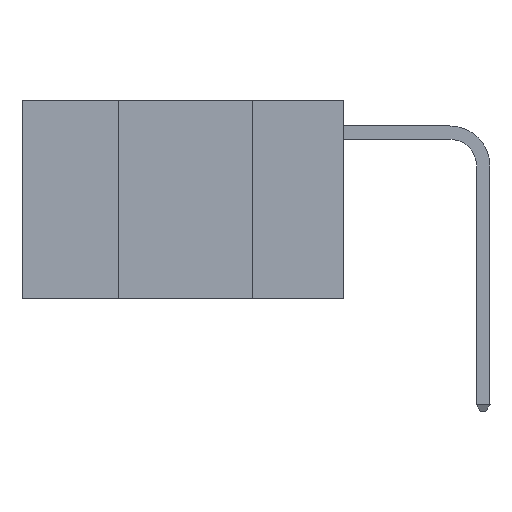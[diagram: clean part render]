
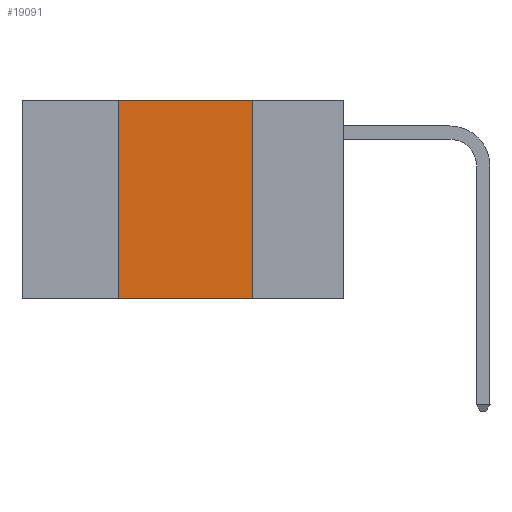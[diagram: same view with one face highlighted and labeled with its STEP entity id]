
A CAD part, left-side view. The second image highlights one B-rep face of the part: STEP entity #19091.
In plain terms, the highlighted planar face has unit normal (-1, 0, 0).
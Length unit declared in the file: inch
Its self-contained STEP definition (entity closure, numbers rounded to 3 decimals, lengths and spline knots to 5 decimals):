
#1354 = CARTESIAN_POINT ( 'NONE',  ( 0., 0.6, 0. ) ) ;
#1694 = CARTESIAN_POINT ( 'NONE',  ( 0., 0.17, 0. ) ) ;
#1809 = AXIS2_PLACEMENT_3D ( 'NONE', #28655, #1908, #17654 ) ;
#1908 = DIRECTION ( 'NONE',  ( 1., 0., 0. ) ) ;
#2780 = VERTEX_POINT ( 'NONE', #6010 ) ;
#4047 = ORIENTED_EDGE ( 'NONE', *, *, #19208, .T. ) ;
#4631 = DIRECTION ( 'NONE',  ( 0., -1., 0. ) ) ;
#4826 = EDGE_CURVE ( 'NONE', #10101, #12527, #15835, .T. ) ;
#5591 = EDGE_CURVE ( 'NONE', #12527, #10860, #24481, .T. ) ;
#6010 = CARTESIAN_POINT ( 'NONE',  ( 0., 0.42, -0.37 ) ) ;
#6105 = DIRECTION ( 'NONE',  ( 0., 0., 1. ) ) ;
#6698 = VECTOR ( 'NONE', #28460, 39.37008 ) ;
#6819 = FACE_OUTER_BOUND ( 'NONE', #18830, .T. ) ;
#8594 = LINE ( 'NONE', #24759, #19745 ) ;
#9740 = VECTOR ( 'NONE', #6105, 39.37008 ) ;
#10101 = VERTEX_POINT ( 'NONE', #16920 ) ;
#10860 = VERTEX_POINT ( 'NONE', #28282 ) ;
#12527 = VERTEX_POINT ( 'NONE', #13823 ) ;
#13823 = CARTESIAN_POINT ( 'NONE',  ( 0., 0.17, 0. ) ) ;
#15140 = VECTOR ( 'NONE', #23710, 39.37008 ) ;
#15427 = PLANE ( 'NONE',  #1809 ) ;
#15835 = LINE ( 'NONE', #1354, #15140 ) ;
#16920 = CARTESIAN_POINT ( 'NONE',  ( 0., 0.42, 0. ) ) ;
#17654 = DIRECTION ( 'NONE',  ( 0., 0., -1. ) ) ;
#18830 = EDGE_LOOP ( 'NONE', ( #20130, #27749, #18947, #4047 ) ) ;
#18947 = ORIENTED_EDGE ( 'NONE', *, *, #22511, .F. ) ;
#19091 = ADVANCED_FACE ( 'NONE', ( #6819 ), #15427, .F. ) ;
#19208 = EDGE_CURVE ( 'NONE', #2780, #10860, #8594, .T. ) ;
#19745 = VECTOR ( 'NONE', #4631, 39.37008 ) ;
#20130 = ORIENTED_EDGE ( 'NONE', *, *, #5591, .F. ) ;
#20872 = LINE ( 'NONE', #26084, #9740 ) ;
#22511 = EDGE_CURVE ( 'NONE', #2780, #10101, #20872, .T. ) ;
#23710 = DIRECTION ( 'NONE',  ( 0., -1., 0. ) ) ;
#24481 = LINE ( 'NONE', #1694, #6698 ) ;
#24759 = CARTESIAN_POINT ( 'NONE',  ( 0., 0.6, -0.37 ) ) ;
#26084 = CARTESIAN_POINT ( 'NONE',  ( 0., 0.42, 0. ) ) ;
#27749 = ORIENTED_EDGE ( 'NONE', *, *, #4826, .F. ) ;
#28282 = CARTESIAN_POINT ( 'NONE',  ( 0., 0.17, -0.37 ) ) ;
#28460 = DIRECTION ( 'NONE',  ( 0., 0., -1. ) ) ;
#28655 = CARTESIAN_POINT ( 'NONE',  ( 0., 0.6, 0. ) ) ;
